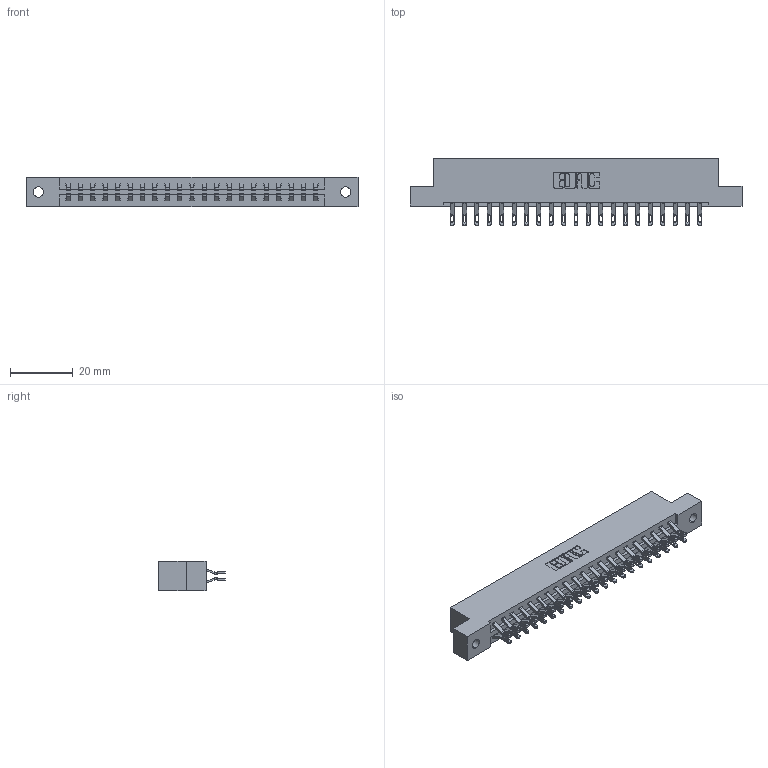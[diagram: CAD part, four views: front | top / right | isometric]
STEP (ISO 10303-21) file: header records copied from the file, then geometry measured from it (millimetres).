
FILE_DESCRIPTION (( 'STEP AP203' ), '1' );
FILE_NAME ('387-042-555-202.STEP', '2018-09-19T23:19:04', ( '' ), ( '' ), 'SwSTEP 2.0', 'SolidWorks 2016', '' );
FILE_SCHEMA (( 'CONFIG_CONTROL_DESIGN' ));
Length unit declared in the file: inch
Products named in the file (3): 337 Part_Flush Mounting Lugs - 0.128 Dia; 345-292-001_555 Tail; 387-042-555-202
Assembly tree (43 placements, depth 2):
  387-042-555-202
    337 Part_Flush Mounting Lugs - 0.128 Dia
    345-292-001_555 Tail  x42
Bounding box: 106.22 x 21.47 x 9.4 mm (x, y, z)
Volume: 11000.2 mm3; surface area: 12418.2 mm2
Topology: 43 solids, 43 shells, 2634 faces, 8249 edges, 5498 vertices
Faces by surface type: plane 1582, cylinder 1052
Entity records: 19327 total; most frequent: CARTESIAN_POINT 3308, ORIENTED_EDGE 3214, DIRECTION 2823, EDGE_CURVE 1607, VECTOR 1459, LINE 1459, VERTEX_POINT 1070, AXIS2_PLACEMENT_3D 682
